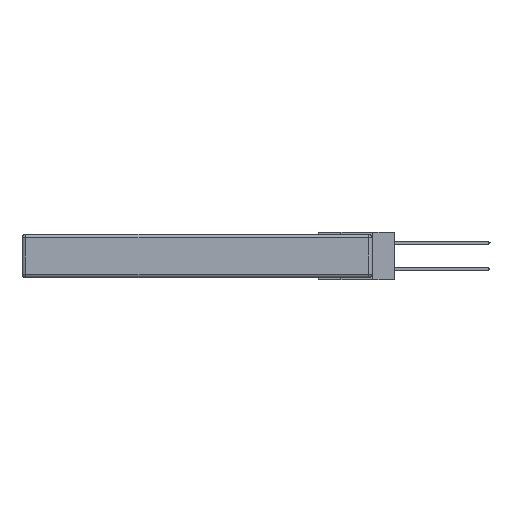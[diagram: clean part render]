
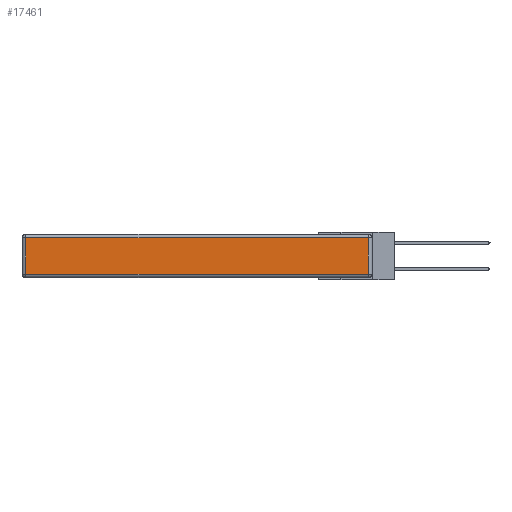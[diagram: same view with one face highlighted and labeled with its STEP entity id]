
A CAD part, left-side view. The second image highlights one B-rep face of the part: STEP entity #17461.
In plain terms, the highlighted planar face has unit normal (-1, 0, 0).
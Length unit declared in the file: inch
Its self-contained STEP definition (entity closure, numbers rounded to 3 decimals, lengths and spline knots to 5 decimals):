
#1204 = DIRECTION ( 'NONE',  ( 0., 0., 1. ) ) ;
#1526 = LINE ( 'NONE', #4047, #8805 ) ;
#2350 = VERTEX_POINT ( 'NONE', #15719 ) ;
#2617 = VECTOR ( 'NONE', #6993, 39.37008 ) ;
#2920 = EDGE_CURVE ( 'NONE', #15001, #15594, #7119, .T. ) ;
#2936 = CARTESIAN_POINT ( 'NONE',  ( 0., 0.03, -0.313 ) ) ;
#3854 = EDGE_CURVE ( 'NONE', #15594, #11155, #17148, .T. ) ;
#4047 = CARTESIAN_POINT ( 'NONE',  ( 0., 2.72, -0.343 ) ) ;
#4540 = DIRECTION ( 'NONE',  ( 0., 1., 0. ) ) ;
#4806 = FACE_OUTER_BOUND ( 'NONE', #19446, .T. ) ;
#6993 = DIRECTION ( 'NONE',  ( 0., -1., 0. ) ) ;
#7119 = LINE ( 'NONE', #15332, #17455 ) ;
#7375 = ORIENTED_EDGE ( 'NONE', *, *, #15006, .T. ) ;
#7560 = ORIENTED_EDGE ( 'NONE', *, *, #21983, .T. ) ;
#7703 = CARTESIAN_POINT ( 'NONE',  ( 0., 0., -0.343 ) ) ;
#7711 = CARTESIAN_POINT ( 'NONE',  ( 0., 2.72, -0.03 ) ) ;
#8805 = VECTOR ( 'NONE', #9385, 39.37008 ) ;
#9284 = DIRECTION ( 'NONE',  ( 0., 0., 1. ) ) ;
#9385 = DIRECTION ( 'NONE',  ( 0., 0., -1. ) ) ;
#9738 = CARTESIAN_POINT ( 'NONE',  ( 0., 2.75, -0.03 ) ) ;
#11155 = VERTEX_POINT ( 'NONE', #7711 ) ;
#11364 = DIRECTION ( 'NONE',  ( -1., 0., 0. ) ) ;
#11491 = ORIENTED_EDGE ( 'NONE', *, *, #2920, .T. ) ;
#12690 = LINE ( 'NONE', #17191, #2617 ) ;
#15001 = VERTEX_POINT ( 'NONE', #2936 ) ;
#15006 = EDGE_CURVE ( 'NONE', #2350, #15001, #12690, .T. ) ;
#15254 = ORIENTED_EDGE ( 'NONE', *, *, #3854, .T. ) ;
#15332 = CARTESIAN_POINT ( 'NONE',  ( 0., 0.03, -0.343 ) ) ;
#15594 = VERTEX_POINT ( 'NONE', #18833 ) ;
#15719 = CARTESIAN_POINT ( 'NONE',  ( 0., 2.72, -0.313 ) ) ;
#16363 = PLANE ( 'NONE',  #16815 ) ;
#16815 = AXIS2_PLACEMENT_3D ( 'NONE', #7703, #11364, #9284 ) ;
#17148 = LINE ( 'NONE', #9738, #20068 ) ;
#17191 = CARTESIAN_POINT ( 'NONE',  ( 0., 0., -0.313 ) ) ;
#17455 = VECTOR ( 'NONE', #1204, 39.37008 ) ;
#17461 = ADVANCED_FACE ( 'NONE', ( #4806 ), #16363, .T. ) ;
#18833 = CARTESIAN_POINT ( 'NONE',  ( 0., 0.03, -0.03 ) ) ;
#19446 = EDGE_LOOP ( 'NONE', ( #7375, #11491, #15254, #7560 ) ) ;
#20068 = VECTOR ( 'NONE', #4540, 39.37008 ) ;
#21983 = EDGE_CURVE ( 'NONE', #11155, #2350, #1526, .T. ) ;
